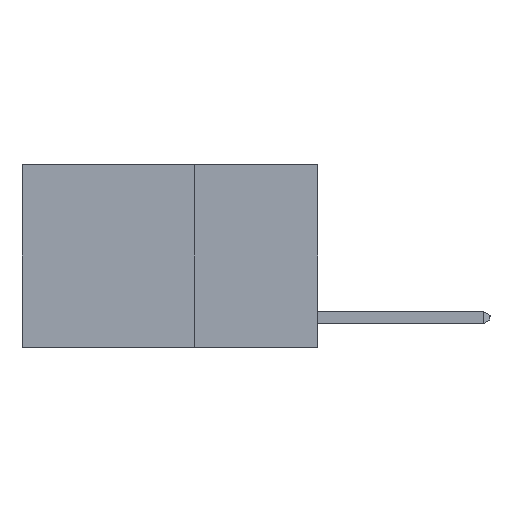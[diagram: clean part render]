
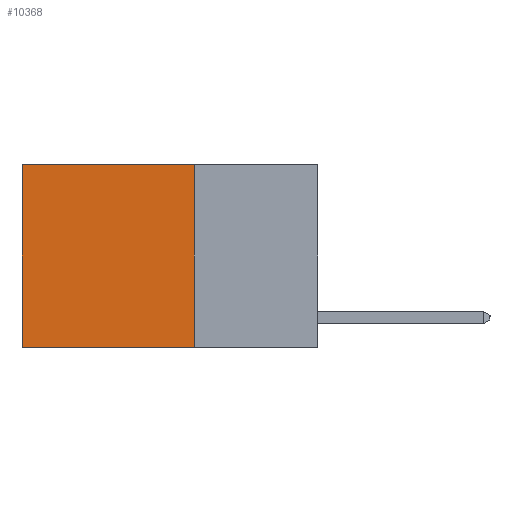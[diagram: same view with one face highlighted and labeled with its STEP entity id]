
A CAD part, left-side view. The second image highlights one B-rep face of the part: STEP entity #10368.
In plain terms, the highlighted planar face has unit normal (-1, 0, 0).
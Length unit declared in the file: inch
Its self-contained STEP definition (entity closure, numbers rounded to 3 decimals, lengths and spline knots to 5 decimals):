
#431 = CARTESIAN_POINT ( 'NONE',  ( 0.2625, 0.25, 0. ) ) ;
#1362 = ORIENTED_EDGE ( 'NONE', *, *, #5347, .T. ) ;
#1416 = DIRECTION ( 'NONE',  ( 0., 0., -1. ) ) ;
#1831 = DIRECTION ( 'NONE',  ( 0., 1., 0. ) ) ;
#2137 = VERTEX_POINT ( 'NONE', #14855 ) ;
#2252 = FACE_OUTER_BOUND ( 'NONE', #5344, .T. ) ;
#2603 = DIRECTION ( 'NONE',  ( 1., 0., 0. ) ) ;
#2908 = CARTESIAN_POINT ( 'NONE',  ( 0.2625, 0.25, 0. ) ) ;
#3000 = LINE ( 'NONE', #16059, #16481 ) ;
#3297 = VECTOR ( 'NONE', #1831, 39.37008 ) ;
#4123 = VECTOR ( 'NONE', #9435, 39.37008 ) ;
#5306 = CARTESIAN_POINT ( 'NONE',  ( 0.2625, 0.25, 0. ) ) ;
#5344 = EDGE_LOOP ( 'NONE', ( #9391, #6617, #8031, #1362 ) ) ;
#5347 = EDGE_CURVE ( 'NONE', #13040, #2137, #13789, .T. ) ;
#5730 = EDGE_CURVE ( 'NONE', #13040, #11188, #11222, .T. ) ;
#6617 = ORIENTED_EDGE ( 'NONE', *, *, #13096, .F. ) ;
#6796 = VECTOR ( 'NONE', #1416, 39.37008 ) ;
#8029 = PLANE ( 'NONE',  #16867 ) ;
#8031 = ORIENTED_EDGE ( 'NONE', *, *, #5730, .F. ) ;
#9305 = CARTESIAN_POINT ( 'NONE',  ( 0.2625, 0.25, 0. ) ) ;
#9391 = ORIENTED_EDGE ( 'NONE', *, *, #14147, .T. ) ;
#9435 = DIRECTION ( 'NONE',  ( 0., 0., -1. ) ) ;
#10368 = ADVANCED_FACE ( 'NONE', ( #2252 ), #8029, .F. ) ;
#10845 = CARTESIAN_POINT ( 'NONE',  ( 0.2625, 0.6, 0. ) ) ;
#10995 = CARTESIAN_POINT ( 'NONE',  ( 0.2625, 0.6, -0.37 ) ) ;
#11188 = VERTEX_POINT ( 'NONE', #13707 ) ;
#11222 = LINE ( 'NONE', #5306, #4123 ) ;
#11932 = DIRECTION ( 'NONE',  ( 0., 0., -1. ) ) ;
#12281 = VERTEX_POINT ( 'NONE', #10995 ) ;
#13040 = VERTEX_POINT ( 'NONE', #2908 ) ;
#13096 = EDGE_CURVE ( 'NONE', #11188, #12281, #3000, .T. ) ;
#13707 = CARTESIAN_POINT ( 'NONE',  ( 0.2625, 0.25, -0.37 ) ) ;
#13789 = LINE ( 'NONE', #431, #3297 ) ;
#14147 = EDGE_CURVE ( 'NONE', #2137, #12281, #16645, .T. ) ;
#14855 = CARTESIAN_POINT ( 'NONE',  ( 0.2625, 0.6, 0. ) ) ;
#16059 = CARTESIAN_POINT ( 'NONE',  ( 0.2625, 0.25, -0.37 ) ) ;
#16114 = DIRECTION ( 'NONE',  ( 0., 1., 0. ) ) ;
#16481 = VECTOR ( 'NONE', #16114, 39.37008 ) ;
#16645 = LINE ( 'NONE', #10845, #6796 ) ;
#16867 = AXIS2_PLACEMENT_3D ( 'NONE', #9305, #2603, #11932 ) ;
